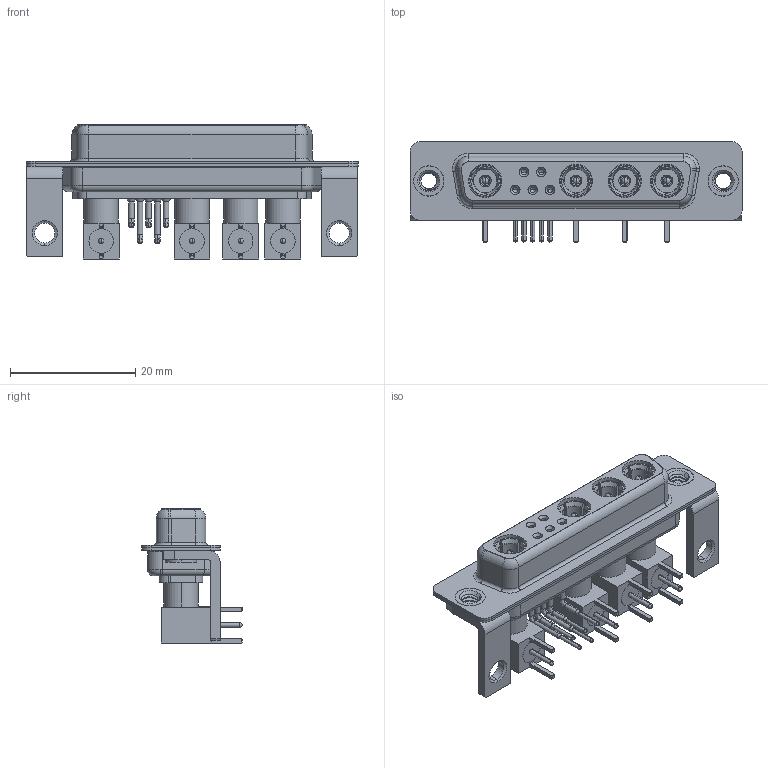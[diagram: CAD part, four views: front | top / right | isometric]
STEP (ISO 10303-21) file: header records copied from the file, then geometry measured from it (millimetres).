
FILE_DESCRIPTION (( 'STEP AP203' ), '1' );
FILE_NAME ('630-9W4-640-7NC.STEP', '2022-06-01T09:41:38', ( '' ), ( '' ), 'SwSTEP 2.0', 'SolidWorks 2020', '' );
FILE_SCHEMA (( 'CONFIG_CONTROL_DESIGN' ));
Length unit declared in the file: millimetre
Products named in the file (18): 630Combo Threaded Rivet_B; Pin_RA; Co-Ax Plug_RA PC Tail; Co-Ax Plug Assy_RA; 630Combo Contact Row 1; 630Combo Contact Row 2; Insulator Pin_Straight PC Tail; 630Combo Shell Rear_25 Contacts; RA Back Shell; 630Combo Housing_9W4; Locking Collar; Insulator RA Pin; 630Combo Shell Front_25 Contacts; 630Combo Stabilizer Bracket; 630-9W4-640-7NC
Assembly tree (40 placements, depth 3):
  630-9W4-640-7NC
    630Combo Housing_9W4
    630Combo Shell Front_25 Contacts
    630Combo Shell Rear_25 Contacts
    630Combo Threaded Rivet_B  x2
    630Combo Stabilizer Bracket  x2
    Co-Ax Plug Assy_RA
      Co-Ax Plug_RA PC Tail
      Insulator Pin_Straight PC Tail
      Pin_RA
      Locking Collar
      RA Back Shell
      Insulator RA Pin
    Co-Ax Plug Assy_RA
      Co-Ax Plug_RA PC Tail
      Insulator Pin_Straight PC Tail
      Pin_RA
      Locking Collar
      RA Back Shell
      Insulator RA Pin
    Co-Ax Plug Assy_RA
      Co-Ax Plug_RA PC Tail
      Insulator Pin_Straight PC Tail
      Pin_RA
      Locking Collar
      RA Back Shell
      Insulator RA Pin
    Co-Ax Plug Assy_RA
      Co-Ax Plug_RA PC Tail
      Insulator Pin_Straight PC Tail
      Pin_RA
      Locking Collar
      RA Back Shell
      Insulator RA Pin
    630Combo Contact Row 1  x2
    630Combo Contact Row 2  x3
Bounding box: 53.05 x 16 x 21.41 mm (x, y, z)
Volume: 4948.1 mm3; surface area: 11919.4 mm2
Topology: 36 solids, 36 shells, 1254 faces, 3064 edges, 1922 vertices
Faces by surface type: cylinder 530, plane 430, cone 167, torus 81, bspline 30, sphere 16
Entity records: 21886 total; most frequent: CARTESIAN_POINT 4981, DIRECTION 3271, ORIENTED_EDGE 2850, EDGE_CURVE 1425, AXIS2_PLACEMENT_3D 1329, VERTEX_POINT 905, CIRCLE 701, EDGE_LOOP 684
